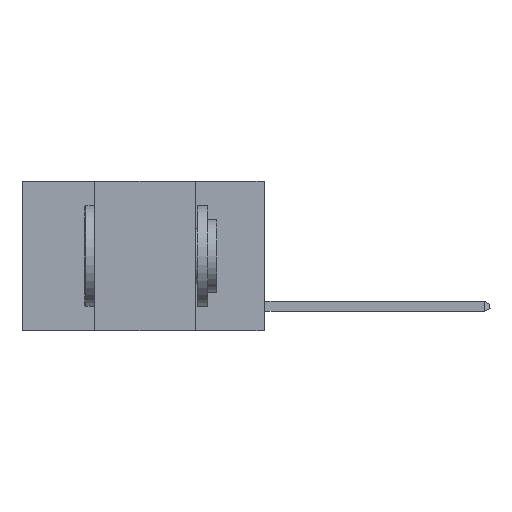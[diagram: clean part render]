
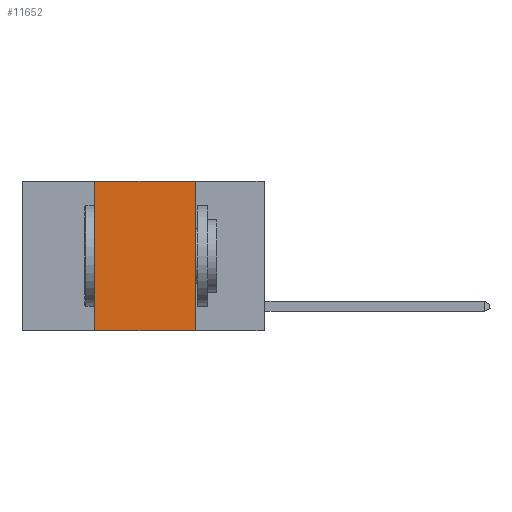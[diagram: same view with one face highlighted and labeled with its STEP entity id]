
A CAD part, left-side view. The second image highlights one B-rep face of the part: STEP entity #11652.
In plain terms, the highlighted planar face has unit normal (-1, 0, 0).
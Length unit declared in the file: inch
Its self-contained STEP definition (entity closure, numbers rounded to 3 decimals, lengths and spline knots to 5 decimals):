
#222 = ORIENTED_EDGE ( 'NONE', *, *, #12819, .F. ) ;
#290 = LINE ( 'NONE', #3936, #12082 ) ;
#879 = AXIS2_PLACEMENT_3D ( 'NONE', #8383, #12469, #962 ) ;
#962 = DIRECTION ( 'NONE',  ( 0., 0., -1. ) ) ;
#1230 = VERTEX_POINT ( 'NONE', #13240 ) ;
#1400 = DIRECTION ( 'NONE',  ( 0., -1., 0. ) ) ;
#1643 = CARTESIAN_POINT ( 'NONE',  ( 0., 0.17, 0. ) ) ;
#1785 = LINE ( 'NONE', #9525, #1896 ) ;
#1896 = VECTOR ( 'NONE', #12116, 39.37008 ) ;
#2321 = FACE_OUTER_BOUND ( 'NONE', #7311, .T. ) ;
#3426 = PLANE ( 'NONE',  #879 ) ;
#3541 = VERTEX_POINT ( 'NONE', #15638 ) ;
#3936 = CARTESIAN_POINT ( 'NONE',  ( 0., 0.6, 0. ) ) ;
#4649 = VERTEX_POINT ( 'NONE', #7591 ) ;
#4864 = ORIENTED_EDGE ( 'NONE', *, *, #14717, .T. ) ;
#7311 = EDGE_LOOP ( 'NONE', ( #10553, #7719, #222, #4864 ) ) ;
#7591 = CARTESIAN_POINT ( 'NONE',  ( 0., 0.42, -0.37 ) ) ;
#7708 = LINE ( 'NONE', #11812, #15562 ) ;
#7719 = ORIENTED_EDGE ( 'NONE', *, *, #9414, .F. ) ;
#7984 = CARTESIAN_POINT ( 'NONE',  ( 0., 0.42, 0. ) ) ;
#8383 = CARTESIAN_POINT ( 'NONE',  ( 0., 0.6, 0. ) ) ;
#9414 = EDGE_CURVE ( 'NONE', #1230, #14191, #290, .T. ) ;
#9525 = CARTESIAN_POINT ( 'NONE',  ( 0., 0.6, -0.37 ) ) ;
#10553 = ORIENTED_EDGE ( 'NONE', *, *, #14124, .F. ) ;
#11652 = ADVANCED_FACE ( 'NONE', ( #2321 ), #3426, .F. ) ;
#11812 = CARTESIAN_POINT ( 'NONE',  ( 0., 0.17, 0. ) ) ;
#11838 = LINE ( 'NONE', #7984, #16372 ) ;
#12082 = VECTOR ( 'NONE', #1400, 39.37008 ) ;
#12116 = DIRECTION ( 'NONE',  ( 0., -1., 0. ) ) ;
#12469 = DIRECTION ( 'NONE',  ( 1., 0., 0. ) ) ;
#12819 = EDGE_CURVE ( 'NONE', #4649, #1230, #11838, .T. ) ;
#13240 = CARTESIAN_POINT ( 'NONE',  ( 0., 0.42, 0. ) ) ;
#14124 = EDGE_CURVE ( 'NONE', #14191, #3541, #7708, .T. ) ;
#14191 = VERTEX_POINT ( 'NONE', #1643 ) ;
#14717 = EDGE_CURVE ( 'NONE', #4649, #3541, #1785, .T. ) ;
#15562 = VECTOR ( 'NONE', #15590, 39.37008 ) ;
#15590 = DIRECTION ( 'NONE',  ( 0., 0., -1. ) ) ;
#15638 = CARTESIAN_POINT ( 'NONE',  ( 0., 0.17, -0.37 ) ) ;
#15773 = DIRECTION ( 'NONE',  ( 0., 0., 1. ) ) ;
#16372 = VECTOR ( 'NONE', #15773, 39.37008 ) ;
